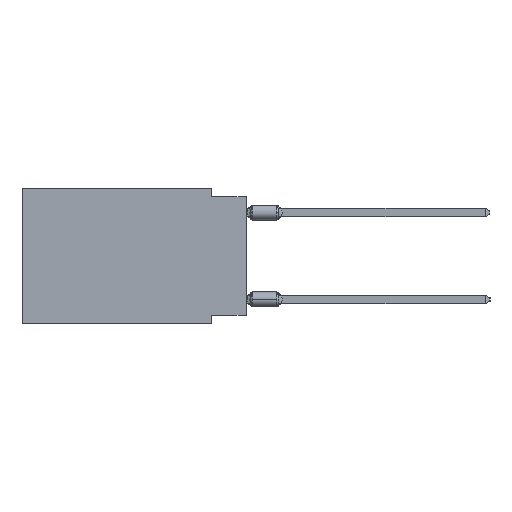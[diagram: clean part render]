
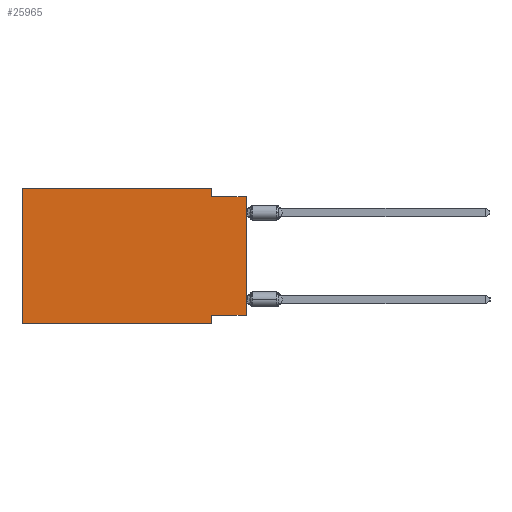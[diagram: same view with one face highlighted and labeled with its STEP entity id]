
A CAD part, left-side view. The second image highlights one B-rep face of the part: STEP entity #25965.
In plain terms, the highlighted planar face has unit normal (-1, 0, 0).
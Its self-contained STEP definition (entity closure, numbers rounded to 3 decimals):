
#142 = CARTESIAN_POINT ( 'NONE',  ( 0., 0., -9.271 ) ) ;
#1102 = DIRECTION ( 'NONE',  ( 0., 0., -1. ) ) ;
#1225 = EDGE_CURVE ( 'NONE', #37121, #32431, #2006, .T. ) ;
#1504 = VECTOR ( 'NONE', #21228, 1000. ) ;
#2006 = LINE ( 'NONE', #5902, #26356 ) ;
#2743 = EDGE_CURVE ( 'NONE', #37121, #21697, #8694, .T. ) ;
#3939 = ORIENTED_EDGE ( 'NONE', *, *, #1225, .T. ) ;
#4599 = CARTESIAN_POINT ( 'NONE',  ( 0., 16.383, 0. ) ) ;
#5022 = AXIS2_PLACEMENT_3D ( 'NONE', #11852, #28790, #1102 ) ;
#5902 = CARTESIAN_POINT ( 'NONE',  ( 0., 16.383, -9.906 ) ) ;
#6284 = CARTESIAN_POINT ( 'NONE',  ( 0., 16.383, 0. ) ) ;
#6906 = CARTESIAN_POINT ( 'NONE',  ( 0., 2.54, -9.906 ) ) ;
#8347 = VERTEX_POINT ( 'NONE', #10286 ) ;
#8694 = LINE ( 'NONE', #4599, #19144 ) ;
#9242 = CARTESIAN_POINT ( 'NONE',  ( 0., 0., -9.271 ) ) ;
#9464 = DIRECTION ( 'NONE',  ( 0., 1., 0. ) ) ;
#9605 = CARTESIAN_POINT ( 'NONE',  ( 0., 2.54, -9.906 ) ) ;
#10286 = CARTESIAN_POINT ( 'NONE',  ( 0., 2.54, -0.635 ) ) ;
#10291 = VERTEX_POINT ( 'NONE', #23685 ) ;
#11852 = CARTESIAN_POINT ( 'NONE',  ( 0., 16.383, 0. ) ) ;
#12478 = VERTEX_POINT ( 'NONE', #142 ) ;
#12888 = CARTESIAN_POINT ( 'NONE',  ( 0., 16.383, -9.906 ) ) ;
#13002 = CARTESIAN_POINT ( 'NONE',  ( 0., 0., -0.635 ) ) ;
#13362 = LINE ( 'NONE', #38495, #29296 ) ;
#13632 = EDGE_CURVE ( 'NONE', #8347, #23264, #41150, .T. ) ;
#14358 = CARTESIAN_POINT ( 'NONE',  ( 0., 2.54, 0. ) ) ;
#15723 = FACE_OUTER_BOUND ( 'NONE', #39005, .T. ) ;
#19144 = VECTOR ( 'NONE', #22204, 1000. ) ;
#19816 = ORIENTED_EDGE ( 'NONE', *, *, #27395, .F. ) ;
#21112 = DIRECTION ( 'NONE',  ( 0., 0., 1. ) ) ;
#21228 = DIRECTION ( 'NONE',  ( 0., 0., -1. ) ) ;
#21697 = VERTEX_POINT ( 'NONE', #26859 ) ;
#21706 = EDGE_CURVE ( 'NONE', #12478, #23264, #13362, .T. ) ;
#21956 = CARTESIAN_POINT ( 'NONE',  ( 0., 0., -0.635 ) ) ;
#22204 = DIRECTION ( 'NONE',  ( 0., 0., 1. ) ) ;
#22837 = DIRECTION ( 'NONE',  ( 0., -1., 0. ) ) ;
#23264 = VERTEX_POINT ( 'NONE', #21956 ) ;
#23685 = CARTESIAN_POINT ( 'NONE',  ( 0., 2.54, -9.271 ) ) ;
#25965 = ADVANCED_FACE ( 'NONE', ( #15723 ), #43616, .F. ) ;
#26356 = VECTOR ( 'NONE', #22837, 1000. ) ;
#26417 = ORIENTED_EDGE ( 'NONE', *, *, #39431, .F. ) ;
#26859 = CARTESIAN_POINT ( 'NONE',  ( 0., 16.383, 0. ) ) ;
#27395 = EDGE_CURVE ( 'NONE', #28927, #8347, #35857, .T. ) ;
#28597 = VECTOR ( 'NONE', #9464, 1000. ) ;
#28790 = DIRECTION ( 'NONE',  ( 1., 0., 0. ) ) ;
#28927 = VERTEX_POINT ( 'NONE', #44520 ) ;
#29296 = VECTOR ( 'NONE', #21112, 1000. ) ;
#29453 = VECTOR ( 'NONE', #38045, 1000. ) ;
#30404 = DIRECTION ( 'NONE',  ( 0., -1., 0. ) ) ;
#30652 = ORIENTED_EDGE ( 'NONE', *, *, #13632, .F. ) ;
#31167 = LINE ( 'NONE', #9242, #28597 ) ;
#32431 = VERTEX_POINT ( 'NONE', #9605 ) ;
#33297 = EDGE_CURVE ( 'NONE', #10291, #32431, #38446, .T. ) ;
#35010 = ORIENTED_EDGE ( 'NONE', *, *, #21706, .T. ) ;
#35857 = LINE ( 'NONE', #14358, #1504 ) ;
#35881 = VECTOR ( 'NONE', #38672, 1000. ) ;
#36430 = ORIENTED_EDGE ( 'NONE', *, *, #33297, .F. ) ;
#37121 = VERTEX_POINT ( 'NONE', #12888 ) ;
#37607 = LINE ( 'NONE', #6284, #29453 ) ;
#38045 = DIRECTION ( 'NONE',  ( 0., -1., 0. ) ) ;
#38446 = LINE ( 'NONE', #6906, #35881 ) ;
#38495 = CARTESIAN_POINT ( 'NONE',  ( 0., 0., 0. ) ) ;
#38672 = DIRECTION ( 'NONE',  ( 0., 0., -1. ) ) ;
#39005 = EDGE_LOOP ( 'NONE', ( #35010, #30652, #19816, #26417, #44656, #3939, #36430, #41173 ) ) ;
#39431 = EDGE_CURVE ( 'NONE', #21697, #28927, #37607, .T. ) ;
#41150 = LINE ( 'NONE', #13002, #43990 ) ;
#41173 = ORIENTED_EDGE ( 'NONE', *, *, #43089, .F. ) ;
#43089 = EDGE_CURVE ( 'NONE', #12478, #10291, #31167, .T. ) ;
#43616 = PLANE ( 'NONE',  #5022 ) ;
#43990 = VECTOR ( 'NONE', #30404, 1000. ) ;
#44520 = CARTESIAN_POINT ( 'NONE',  ( 0., 2.54, 0. ) ) ;
#44656 = ORIENTED_EDGE ( 'NONE', *, *, #2743, .F. ) ;
